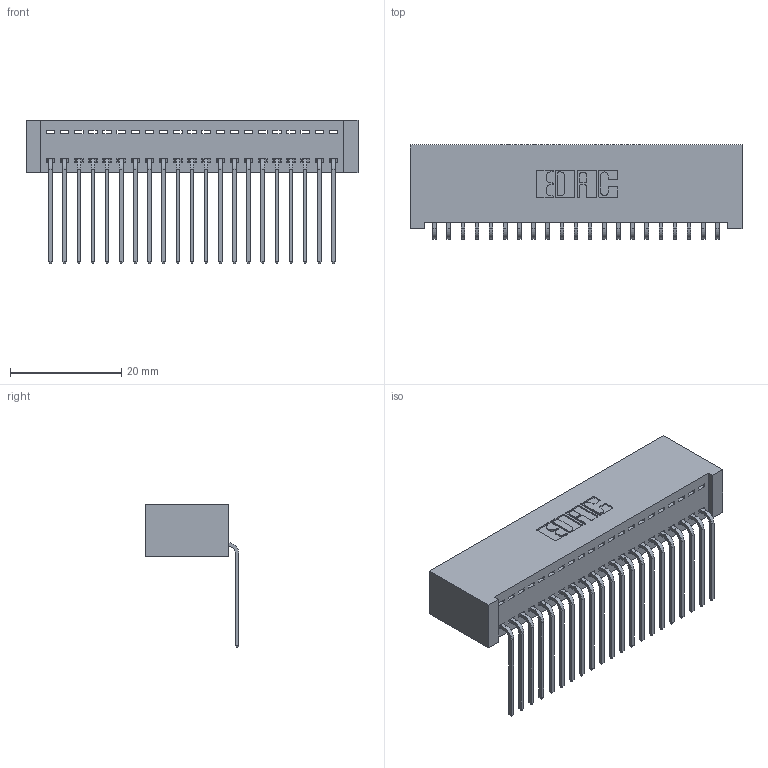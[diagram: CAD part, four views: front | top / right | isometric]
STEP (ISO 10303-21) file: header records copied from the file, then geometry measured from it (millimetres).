
FILE_DESCRIPTION (( 'STEP AP203' ), '1' );
FILE_NAME ('392-021-559-101.STEP', '2018-08-15T12:22:29', ( '' ), ( '' ), 'SwSTEP 2.0', 'SolidWorks 2016', '' );
FILE_SCHEMA (( 'CONFIG_CONTROL_DESIGN' ));
Length unit declared in the file: inch
Products named in the file (3): 342 Part_Lugless; 345-292-001_558 559 Tail - 1; 392-021-559-101
Assembly tree (22 placements, depth 2):
  392-021-559-101
    342 Part_Lugless
    345-292-001_558 559 Tail - 1  x21
Bounding box: 59.59 x 16.83 x 25.78 mm (x, y, z)
Volume: 5626.3 mm3; surface area: 8590.5 mm2
Topology: 22 solids, 22 shells, 1362 faces, 4097 edges, 2702 vertices
Faces by surface type: plane 986, cylinder 376
Entity records: 15229 total; most frequent: CARTESIAN_POINT 2637, ORIENTED_EDGE 2594, DIRECTION 2259, EDGE_CURVE 1297, LINE 1177, VECTOR 1177, VERTEX_POINT 862, AXIS2_PLACEMENT_3D 541
